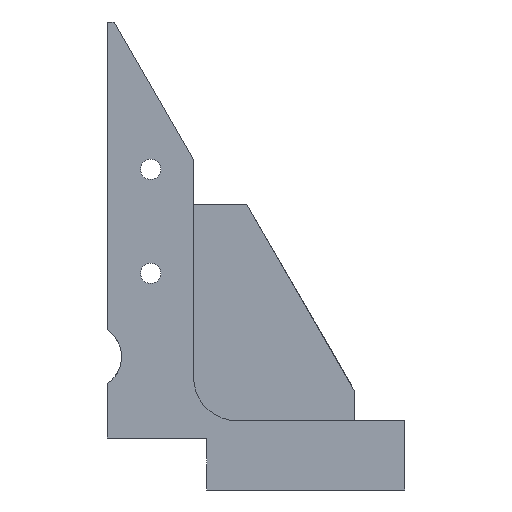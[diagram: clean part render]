
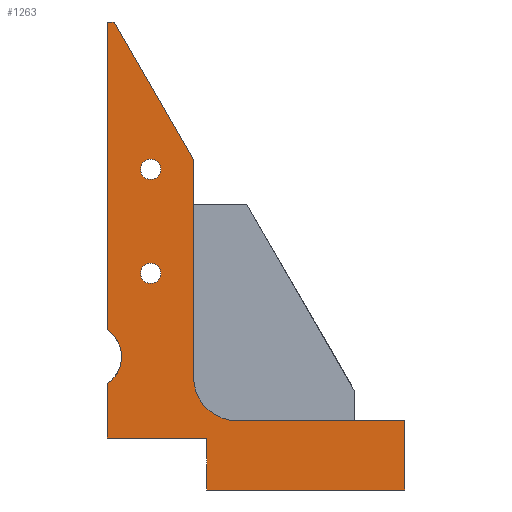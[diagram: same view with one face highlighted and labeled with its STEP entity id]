
A CAD part, left-side view. The second image highlights one B-rep face of the part: STEP entity #1263.
In plain terms, the highlighted planar face has unit normal (-1, 0, 0).
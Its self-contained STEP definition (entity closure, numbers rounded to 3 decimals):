
#3 = VERTEX_POINT ( 'NONE', #1380 ) ;
#36 = LINE ( 'NONE', #383, #1879 ) ;
#68 = LINE ( 'NONE', #2196, #1916 ) ;
#78 = ORIENTED_EDGE ( 'NONE', *, *, #1736, .T. ) ;
#103 = VERTEX_POINT ( 'NONE', #867 ) ;
#125 = CARTESIAN_POINT ( 'NONE',  ( -8.763, 30.931, 16.51 ) ) ;
#132 = EDGE_CURVE ( 'NONE', #889, #3, #1504, .T. ) ;
#139 = ORIENTED_EDGE ( 'NONE', *, *, #1494, .T. ) ;
#143 = CIRCLE ( 'NONE', #972, 4.763 ) ;
#167 = ORIENTED_EDGE ( 'NONE', *, *, #1808, .T. ) ;
#203 = DIRECTION ( 'NONE',  ( 1., 0., 0. ) ) ;
#205 = EDGE_LOOP ( 'NONE', ( #217, #167 ) ) ;
#217 = ORIENTED_EDGE ( 'NONE', *, *, #1440, .T. ) ;
#226 = AXIS2_PLACEMENT_3D ( 'NONE', #1496, #419, #1667 ) ;
#231 = CARTESIAN_POINT ( 'NONE',  ( -8.763, 37.211, 45.49 ) ) ;
#267 = ORIENTED_EDGE ( 'NONE', *, *, #2038, .T. ) ;
#284 = FACE_BOUND ( 'NONE', #714, .T. ) ;
#293 = EDGE_LOOP ( 'NONE', ( #1059, #1892, #2321, #1786, #825, #861, #2030, #78, #139, #436, #2231, #753 ) ) ;
#316 = DIRECTION ( 'NONE',  ( 0., 1., 0. ) ) ;
#319 = EDGE_CURVE ( 'NONE', #1282, #1895, #1659, .T. ) ;
#327 = CARTESIAN_POINT ( 'NONE',  ( -8.763, 42.545, 68.58 ) ) ;
#343 = CARTESIAN_POINT ( 'NONE',  ( -8.763, 29.026, 7.62 ) ) ;
#366 = PLANE ( 'NONE',  #1706 ) ;
#368 = EDGE_CURVE ( 'NONE', #1112, #889, #1082, .T. ) ;
#374 = CARTESIAN_POINT ( 'NONE',  ( -8.763, 29.026, 0. ) ) ;
#383 = CARTESIAN_POINT ( 'NONE',  ( -8.763, 0., 7.62 ) ) ;
#388 = DIRECTION ( 'NONE',  ( 1., 0., 0. ) ) ;
#415 = VERTEX_POINT ( 'NONE', #870 ) ;
#419 = DIRECTION ( 'NONE',  ( 1., 0., 0. ) ) ;
#436 = ORIENTED_EDGE ( 'NONE', *, *, #1258, .T. ) ;
#497 = AXIS2_PLACEMENT_3D ( 'NONE', #905, #2158, #1088 ) ;
#517 = DIRECTION ( 'NONE',  ( 0., 0., -1. ) ) ;
#552 = DIRECTION ( 'NONE',  ( 0., 0., -1. ) ) ;
#554 = CIRCLE ( 'NONE', #1348, 6.35 ) ;
#590 = CIRCLE ( 'NONE', #1383, 1.5 ) ;
#600 = CARTESIAN_POINT ( 'NONE',  ( -8.763, 0., 10.16 ) ) ;
#608 = EDGE_CURVE ( 'NONE', #823, #1112, #1521, .T. ) ;
#629 = DIRECTION ( 'NONE',  ( 1., 0., 0. ) ) ;
#658 = DIRECTION ( 'NONE',  ( 0., -1., 0. ) ) ;
#659 = VECTOR ( 'NONE', #316, 1000. ) ;
#667 = VERTEX_POINT ( 'NONE', #1767 ) ;
#714 = EDGE_LOOP ( 'NONE', ( #1697, #267 ) ) ;
#719 = VECTOR ( 'NONE', #658, 1000. ) ;
#743 = CIRCLE ( 'NONE', #1152, 1.5 ) ;
#745 = EDGE_CURVE ( 'NONE', #1895, #2179, #1248, .T. ) ;
#753 = ORIENTED_EDGE ( 'NONE', *, *, #745, .T. ) ;
#763 = DIRECTION ( 'NONE',  ( 0., -1., 0. ) ) ;
#823 = VERTEX_POINT ( 'NONE', #1123 ) ;
#825 = ORIENTED_EDGE ( 'NONE', *, *, #368, .T. ) ;
#831 = VERTEX_POINT ( 'NONE', #231 ) ;
#836 = VERTEX_POINT ( 'NONE', #1839 ) ;
#845 = EDGE_CURVE ( 'NONE', #943, #823, #68, .T. ) ;
#853 = DIRECTION ( 'NONE',  ( 1., 0., 0. ) ) ;
#861 = ORIENTED_EDGE ( 'NONE', *, *, #132, .T. ) ;
#862 = DIRECTION ( 'NONE',  ( 0., 0.5, 0.866 ) ) ;
#867 = CARTESIAN_POINT ( 'NONE',  ( -8.763, 37.211, 30.25 ) ) ;
#870 = CARTESIAN_POINT ( 'NONE',  ( -8.763, 37.211, 48.49 ) ) ;
#889 = VERTEX_POINT ( 'NONE', #1317 ) ;
#905 = CARTESIAN_POINT ( 'NONE',  ( -8.763, 37.211, 46.99 ) ) ;
#938 = DIRECTION ( 'NONE',  ( 0., 1., 0. ) ) ;
#943 = VERTEX_POINT ( 'NONE', #125 ) ;
#963 = CARTESIAN_POINT ( 'NONE',  ( -8.763, 24.581, 10.16 ) ) ;
#967 = VECTOR ( 'NONE', #517, 1000. ) ;
#972 = AXIS2_PLACEMENT_3D ( 'NONE', #1274, #203, #1457 ) ;
#1011 = EDGE_CURVE ( 'NONE', #415, #831, #743, .T. ) ;
#1059 = ORIENTED_EDGE ( 'NONE', *, *, #1574, .T. ) ;
#1082 = LINE ( 'NONE', #1398, #659 ) ;
#1088 = DIRECTION ( 'NONE',  ( 0., 0., -1. ) ) ;
#1094 = DIRECTION ( 'NONE',  ( 0., 0., -1. ) ) ;
#1098 = CIRCLE ( 'NONE', #497, 1.5 ) ;
#1107 = VECTOR ( 'NONE', #862, 1000. ) ;
#1112 = VERTEX_POINT ( 'NONE', #327 ) ;
#1123 = CARTESIAN_POINT ( 'NONE',  ( -8.763, 30.931, 48.463 ) ) ;
#1127 = FACE_OUTER_BOUND ( 'NONE', #293, .T. ) ;
#1152 = AXIS2_PLACEMENT_3D ( 'NONE', #1936, #853, #2102 ) ;
#1175 = CARTESIAN_POINT ( 'NONE',  ( -8.763, 43.561, 0. ) ) ;
#1182 = LINE ( 'NONE', #1268, #2070 ) ;
#1201 = VERTEX_POINT ( 'NONE', #343 ) ;
#1248 = LINE ( 'NONE', #1447, #1655 ) ;
#1258 = EDGE_CURVE ( 'NONE', #1201, #1282, #1182, .T. ) ;
#1263 = ADVANCED_FACE ( 'NONE', ( #284, #1611, #1127 ), #366, .F. ) ;
#1268 = CARTESIAN_POINT ( 'NONE',  ( -8.763, 29.026, 0. ) ) ;
#1269 = DIRECTION ( 'NONE',  ( 0., 0., 1. ) ) ;
#1274 = CARTESIAN_POINT ( 'NONE',  ( -8.763, 46.228, 19.533 ) ) ;
#1282 = VERTEX_POINT ( 'NONE', #374 ) ;
#1289 = LINE ( 'NONE', #1175, #2183 ) ;
#1310 = DIRECTION ( 'NONE',  ( 0., 0., 1. ) ) ;
#1317 = CARTESIAN_POINT ( 'NONE',  ( -8.763, 43.561, 68.58 ) ) ;
#1326 = EDGE_CURVE ( 'NONE', #2199, #943, #554, .T. ) ;
#1348 = AXIS2_PLACEMENT_3D ( 'NONE', #1466, #388, #1638 ) ;
#1359 = DIRECTION ( 'NONE',  ( 0., 0., -1. ) ) ;
#1380 = CARTESIAN_POINT ( 'NONE',  ( -8.763, 43.561, 23.478 ) ) ;
#1383 = AXIS2_PLACEMENT_3D ( 'NONE', #1696, #629, #1877 ) ;
#1398 = CARTESIAN_POINT ( 'NONE',  ( -8.763, 0., 68.58 ) ) ;
#1440 = EDGE_CURVE ( 'NONE', #1445, #103, #1681, .T. ) ;
#1445 = VERTEX_POINT ( 'NONE', #1851 ) ;
#1447 = CARTESIAN_POINT ( 'NONE',  ( -8.763, 0., 0. ) ) ;
#1457 = DIRECTION ( 'NONE',  ( 0., 0., -1. ) ) ;
#1466 = CARTESIAN_POINT ( 'NONE',  ( -8.763, 24.581, 16.51 ) ) ;
#1494 = EDGE_CURVE ( 'NONE', #836, #1201, #36, .T. ) ;
#1496 = CARTESIAN_POINT ( 'NONE',  ( -8.763, 37.211, 31.75 ) ) ;
#1504 = LINE ( 'NONE', #2304, #967 ) ;
#1521 = LINE ( 'NONE', #2300, #1107 ) ;
#1574 = EDGE_CURVE ( 'NONE', #2179, #2199, #1774, .T. ) ;
#1611 = FACE_BOUND ( 'NONE', #205, .T. ) ;
#1638 = DIRECTION ( 'NONE',  ( 0., 0., -1. ) ) ;
#1655 = VECTOR ( 'NONE', #1269, 1000. ) ;
#1659 = LINE ( 'NONE', #2080, #719 ) ;
#1667 = DIRECTION ( 'NONE',  ( 0., 0., -1. ) ) ;
#1676 = CARTESIAN_POINT ( 'NONE',  ( -8.763, 0., 10.16 ) ) ;
#1681 = CIRCLE ( 'NONE', #226, 1.5 ) ;
#1696 = CARTESIAN_POINT ( 'NONE',  ( -8.763, 37.211, 31.75 ) ) ;
#1697 = ORIENTED_EDGE ( 'NONE', *, *, #1011, .T. ) ;
#1706 = AXIS2_PLACEMENT_3D ( 'NONE', #1981, #2160, #1094 ) ;
#1736 = EDGE_CURVE ( 'NONE', #667, #836, #1289, .T. ) ;
#1767 = CARTESIAN_POINT ( 'NONE',  ( -8.763, 43.561, 15.587 ) ) ;
#1774 = LINE ( 'NONE', #600, #2246 ) ;
#1786 = ORIENTED_EDGE ( 'NONE', *, *, #608, .T. ) ;
#1808 = EDGE_CURVE ( 'NONE', #103, #1445, #590, .T. ) ;
#1839 = CARTESIAN_POINT ( 'NONE',  ( -8.763, 43.561, 7.62 ) ) ;
#1851 = CARTESIAN_POINT ( 'NONE',  ( -8.763, 37.211, 33.25 ) ) ;
#1877 = DIRECTION ( 'NONE',  ( 0., 0., -1. ) ) ;
#1879 = VECTOR ( 'NONE', #763, 1000. ) ;
#1892 = ORIENTED_EDGE ( 'NONE', *, *, #1326, .T. ) ;
#1895 = VERTEX_POINT ( 'NONE', #2247 ) ;
#1916 = VECTOR ( 'NONE', #1310, 1000. ) ;
#1936 = CARTESIAN_POINT ( 'NONE',  ( -8.763, 37.211, 46.99 ) ) ;
#1981 = CARTESIAN_POINT ( 'NONE',  ( -8.763, 0., 0. ) ) ;
#2030 = ORIENTED_EDGE ( 'NONE', *, *, #2084, .T. ) ;
#2038 = EDGE_CURVE ( 'NONE', #831, #415, #1098, .T. ) ;
#2070 = VECTOR ( 'NONE', #552, 1000. ) ;
#2080 = CARTESIAN_POINT ( 'NONE',  ( -8.763, 0., 0. ) ) ;
#2084 = EDGE_CURVE ( 'NONE', #3, #667, #143, .T. ) ;
#2102 = DIRECTION ( 'NONE',  ( 0., 0., -1. ) ) ;
#2158 = DIRECTION ( 'NONE',  ( 1., 0., 0. ) ) ;
#2160 = DIRECTION ( 'NONE',  ( 1., 0., 0. ) ) ;
#2179 = VERTEX_POINT ( 'NONE', #1676 ) ;
#2183 = VECTOR ( 'NONE', #1359, 1000. ) ;
#2196 = CARTESIAN_POINT ( 'NONE',  ( -8.763, 30.931, 0. ) ) ;
#2199 = VERTEX_POINT ( 'NONE', #963 ) ;
#2231 = ORIENTED_EDGE ( 'NONE', *, *, #319, .T. ) ;
#2246 = VECTOR ( 'NONE', #938, 1000. ) ;
#2247 = CARTESIAN_POINT ( 'NONE',  ( -8.763, 0., 0. ) ) ;
#2300 = CARTESIAN_POINT ( 'NONE',  ( -8.763, 2.213, -1.278 ) ) ;
#2304 = CARTESIAN_POINT ( 'NONE',  ( -8.763, 43.561, 0. ) ) ;
#2321 = ORIENTED_EDGE ( 'NONE', *, *, #845, .T. ) ;
